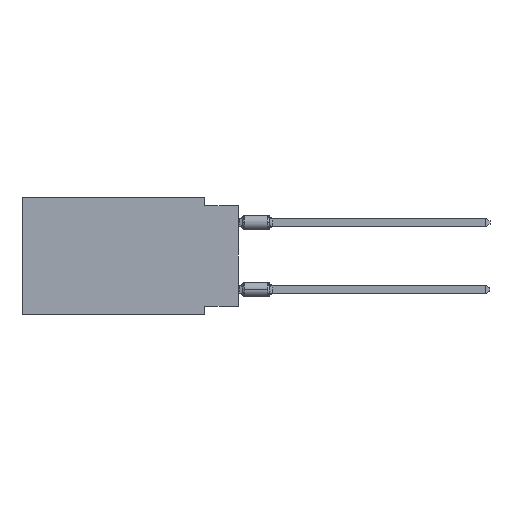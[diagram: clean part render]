
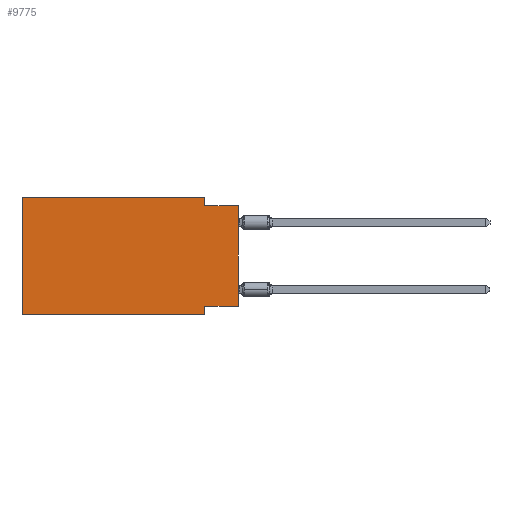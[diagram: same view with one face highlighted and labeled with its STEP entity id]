
A CAD part, left-side view. The second image highlights one B-rep face of the part: STEP entity #9775.
In plain terms, the highlighted planar face has unit normal (-1, 0, 0).
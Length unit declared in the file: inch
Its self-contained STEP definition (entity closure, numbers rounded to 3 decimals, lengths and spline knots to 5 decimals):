
#671 = CARTESIAN_POINT ( 'NONE',  ( 0., 0.1, -0.325 ) ) ;
#714 = VECTOR ( 'NONE', #3213, 39.37008 ) ;
#748 = LINE ( 'NONE', #12426, #714 ) ;
#937 = VERTEX_POINT ( 'NONE', #10837 ) ;
#944 = CARTESIAN_POINT ( 'NONE',  ( 0., 0.645, -0.35 ) ) ;
#1009 = CARTESIAN_POINT ( 'NONE',  ( 0., 0.1, -0.35 ) ) ;
#1025 = ORIENTED_EDGE ( 'NONE', *, *, #7561, .F. ) ;
#1065 = LINE ( 'NONE', #5745, #4710 ) ;
#1087 = DIRECTION ( 'NONE',  ( 0., 0., -1. ) ) ;
#1254 = VERTEX_POINT ( 'NONE', #14408 ) ;
#1973 = CARTESIAN_POINT ( 'NONE',  ( 0., 0.1, 0. ) ) ;
#2021 = ORIENTED_EDGE ( 'NONE', *, *, #7924, .F. ) ;
#2260 = PLANE ( 'NONE',  #14814 ) ;
#2473 = EDGE_CURVE ( 'NONE', #8927, #10315, #4573, .T. ) ;
#2590 = CARTESIAN_POINT ( 'NONE',  ( 0., 0.1, -0.025 ) ) ;
#2880 = EDGE_CURVE ( 'NONE', #8927, #14053, #14949, .T. ) ;
#2974 = CARTESIAN_POINT ( 'NONE',  ( 0., 0.645, 0. ) ) ;
#3213 = DIRECTION ( 'NONE',  ( 0., -1., 0. ) ) ;
#3689 = EDGE_LOOP ( 'NONE', ( #9632, #2021, #13321, #1025, #5346, #8862, #8675, #9013 ) ) ;
#3939 = CARTESIAN_POINT ( 'NONE',  ( 0., 0.1, -0.35 ) ) ;
#4316 = DIRECTION ( 'NONE',  ( 0., -1., 0. ) ) ;
#4367 = LINE ( 'NONE', #10198, #7119 ) ;
#4460 = VECTOR ( 'NONE', #4316, 39.37008 ) ;
#4573 = LINE ( 'NONE', #9250, #14535 ) ;
#4710 = VECTOR ( 'NONE', #10430, 39.37008 ) ;
#5346 = ORIENTED_EDGE ( 'NONE', *, *, #2473, .F. ) ;
#5378 = CARTESIAN_POINT ( 'NONE',  ( 0., 0.645, -0.35 ) ) ;
#5543 = DIRECTION ( 'NONE',  ( 0., 0., -1. ) ) ;
#5745 = CARTESIAN_POINT ( 'NONE',  ( 0., 0., 0. ) ) ;
#6938 = CARTESIAN_POINT ( 'NONE',  ( 0., 0.645, 0. ) ) ;
#7008 = DIRECTION ( 'NONE',  ( 1., 0., 0. ) ) ;
#7119 = VECTOR ( 'NONE', #10124, 39.37008 ) ;
#7561 = EDGE_CURVE ( 'NONE', #10315, #10958, #4367, .T. ) ;
#7924 = EDGE_CURVE ( 'NONE', #12334, #937, #748, .T. ) ;
#7989 = VERTEX_POINT ( 'NONE', #671 ) ;
#8675 = ORIENTED_EDGE ( 'NONE', *, *, #10251, .F. ) ;
#8862 = ORIENTED_EDGE ( 'NONE', *, *, #2880, .T. ) ;
#8927 = VERTEX_POINT ( 'NONE', #5378 ) ;
#9013 = ORIENTED_EDGE ( 'NONE', *, *, #12808, .F. ) ;
#9250 = CARTESIAN_POINT ( 'NONE',  ( 0., 0.645, 0. ) ) ;
#9546 = LINE ( 'NONE', #14247, #10821 ) ;
#9632 = ORIENTED_EDGE ( 'NONE', *, *, #13521, .T. ) ;
#9775 = ADVANCED_FACE ( 'NONE', ( #14237 ), #2260, .F. ) ;
#10124 = DIRECTION ( 'NONE',  ( 0., -1., 0. ) ) ;
#10198 = CARTESIAN_POINT ( 'NONE',  ( 0., 0.645, 0. ) ) ;
#10251 = EDGE_CURVE ( 'NONE', #7989, #14053, #11538, .T. ) ;
#10315 = VERTEX_POINT ( 'NONE', #2974 ) ;
#10430 = DIRECTION ( 'NONE',  ( 0., 0., 1. ) ) ;
#10770 = DIRECTION ( 'NONE',  ( 0., 1., 0. ) ) ;
#10821 = VECTOR ( 'NONE', #10770, 39.37008 ) ;
#10837 = CARTESIAN_POINT ( 'NONE',  ( 0., 0., -0.025 ) ) ;
#10958 = VERTEX_POINT ( 'NONE', #1973 ) ;
#11538 = LINE ( 'NONE', #1009, #14577 ) ;
#11703 = CARTESIAN_POINT ( 'NONE',  ( 0., 0.1, 0. ) ) ;
#12334 = VERTEX_POINT ( 'NONE', #2590 ) ;
#12426 = CARTESIAN_POINT ( 'NONE',  ( 0., 0., -0.025 ) ) ;
#12487 = DIRECTION ( 'NONE',  ( 0., 0., 1. ) ) ;
#12808 = EDGE_CURVE ( 'NONE', #1254, #7989, #9546, .T. ) ;
#13321 = ORIENTED_EDGE ( 'NONE', *, *, #14216, .F. ) ;
#13521 = EDGE_CURVE ( 'NONE', #1254, #937, #1065, .T. ) ;
#13699 = LINE ( 'NONE', #11703, #13828 ) ;
#13828 = VECTOR ( 'NONE', #5543, 39.37008 ) ;
#14053 = VERTEX_POINT ( 'NONE', #3939 ) ;
#14093 = DIRECTION ( 'NONE',  ( 0., 0., -1. ) ) ;
#14216 = EDGE_CURVE ( 'NONE', #10958, #12334, #13699, .T. ) ;
#14237 = FACE_OUTER_BOUND ( 'NONE', #3689, .T. ) ;
#14247 = CARTESIAN_POINT ( 'NONE',  ( 0., 0., -0.325 ) ) ;
#14408 = CARTESIAN_POINT ( 'NONE',  ( 0., 0., -0.325 ) ) ;
#14535 = VECTOR ( 'NONE', #12487, 39.37008 ) ;
#14577 = VECTOR ( 'NONE', #1087, 39.37008 ) ;
#14814 = AXIS2_PLACEMENT_3D ( 'NONE', #6938, #7008, #14093 ) ;
#14949 = LINE ( 'NONE', #944, #4460 ) ;
